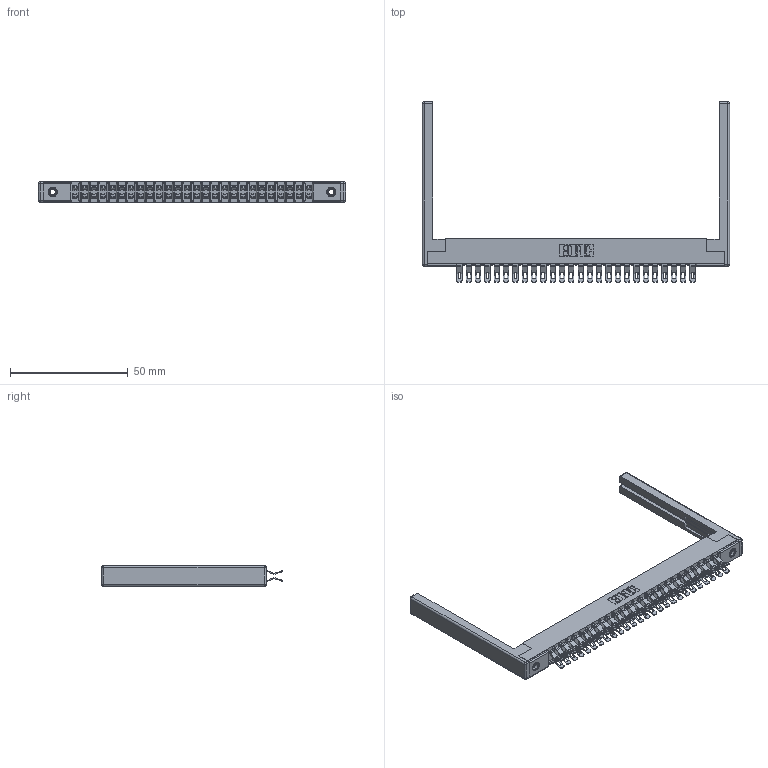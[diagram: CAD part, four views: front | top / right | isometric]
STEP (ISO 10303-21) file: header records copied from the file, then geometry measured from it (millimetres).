
FILE_DESCRIPTION (( 'STEP AP203' ), '1' );
FILE_NAME ('357-052-555-268.STEP', '2019-09-19T03:30:13', ( '' ), ( '' ), 'SwSTEP 2.0', 'SolidWorks 2016', '' );
FILE_SCHEMA (( 'CONFIG_CONTROL_DESIGN' ));
Length unit declared in the file: inch
Products named in the file (5): 307-220-068; 357-052-555-268; 345-250-001_345-250-001-102; 307-290-001_555; 307 Part_.156 Dia Mounting Holes
Assembly tree (57 placements, depth 2):
  357-052-555-268
    307 Part_.156 Dia Mounting Holes
    307-290-001_555  x52
    307-220-068  x2
    345-250-001_345-250-001-102  x2
Bounding box: 130.45 x 76.71 x 8.71 mm (x, y, z)
Volume: 13249.1 mm3; surface area: 20452.6 mm2
Topology: 57 solids, 57 shells, 3471 faces, 10125 edges, 6586 vertices
Faces by surface type: plane 1926, cylinder 1467, sphere 62, cone 12, torus 4
Entity records: 28390 total; most frequent: CARTESIAN_POINT 4631, ORIENTED_EDGE 4582, DIRECTION 4565, EDGE_CURVE 2291, LINE 1737, VECTOR 1737, VERTEX_POINT 1480, AXIS2_PLACEMENT_3D 1414
